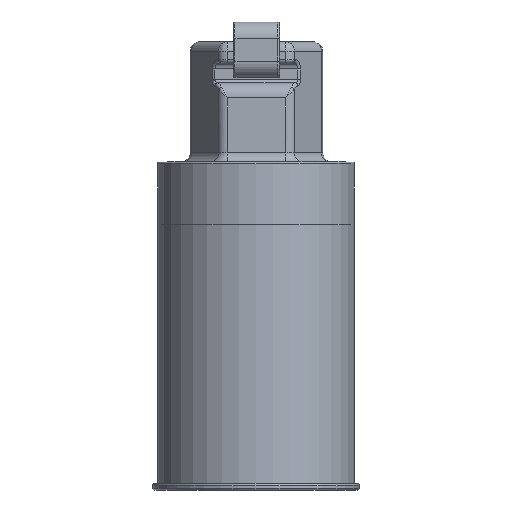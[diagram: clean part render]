
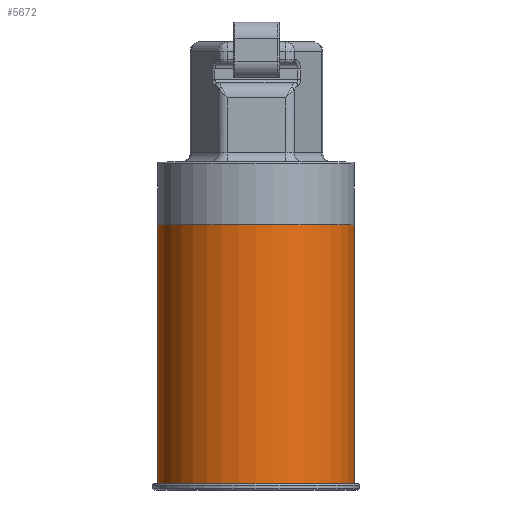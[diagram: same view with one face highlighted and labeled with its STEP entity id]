
A CAD part, left-side view. The second image highlights one B-rep face of the part: STEP entity #5672.
In plain terms, the highlighted cylindrical face has radius 31.5 mm (diameter 63 mm), a full revolution.
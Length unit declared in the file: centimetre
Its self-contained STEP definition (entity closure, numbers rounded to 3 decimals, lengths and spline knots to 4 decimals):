
#951=CYLINDRICAL_SURFACE($,#6084,3.15);
#1205=FACE_BOUND($,#1655,.T.);
#1264=FACE_OUTER_BOUND($,#1654,.T.);
#1654=EDGE_LOOP($,(#3867));
#1655=EDGE_LOOP($,(#3868));
#2087=CIRCLE($,#6082,3.15);
#2088=CIRCLE($,#6085,3.15);
#2450=VERTEX_POINT($,#8688);
#2451=VERTEX_POINT($,#8692);
#2979=EDGE_CURVE($,#2450,#2450,#2087,.T.);
#2980=EDGE_CURVE($,#2451,#2451,#2088,.T.);
#3867=ORIENTED_EDGE($,*,*,#2979,.F.);
#3868=ORIENTED_EDGE($,*,*,#2980,.F.);
#5672=ADVANCED_FACE($,(#1264,#1205),#951,.T.);
#6082=AXIS2_PLACEMENT_3D($,#8689,#6857,#6858);
#6084=AXIS2_PLACEMENT_3D($,#8691,#6861,#6862);
#6085=AXIS2_PLACEMENT_3D($,#8693,#6863,#6864);
#6857=DIRECTION('center_axis',(0.,0.,-1.));
#6858=DIRECTION('ref_axis',(0.,-1.,0.));
#6861=DIRECTION('center_axis',(0.,0.,1.));
#6862=DIRECTION('ref_axis',(0.,1.,0.));
#6863=DIRECTION('center_axis',(0.,0.,1.));
#6864=DIRECTION('ref_axis',(0.,1.,0.));
#8688=CARTESIAN_POINT('',(-1.85,10.,1.85));
#8689=CARTESIAN_POINT('Origin',(-5.,10.,1.85));
#8691=CARTESIAN_POINT('Origin',(-5.,10.,9.));
#8692=CARTESIAN_POINT('',(-5.,6.85,10.15));
#8693=CARTESIAN_POINT('Origin',(-5.,10.,10.15));
